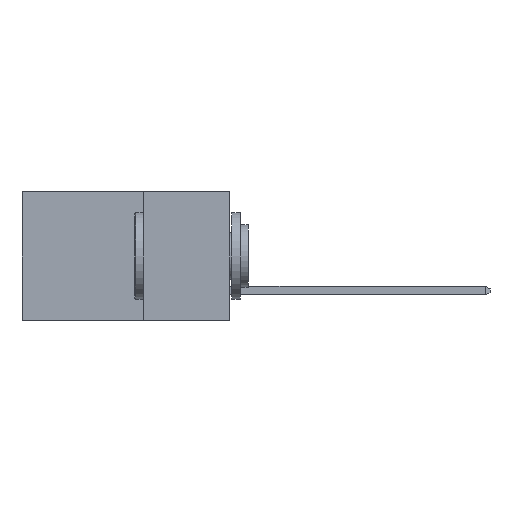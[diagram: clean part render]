
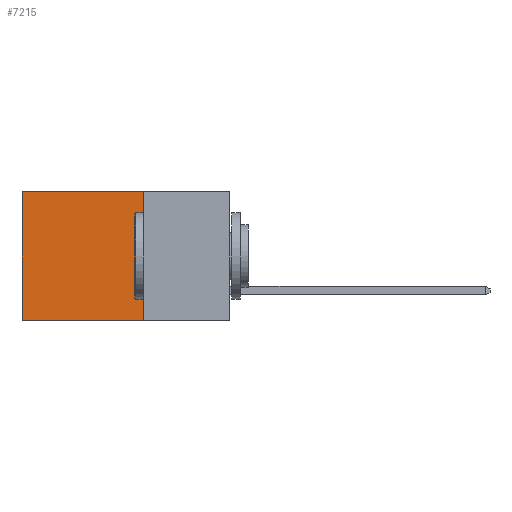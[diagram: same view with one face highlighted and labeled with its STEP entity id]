
A CAD part, left-side view. The second image highlights one B-rep face of the part: STEP entity #7215.
In plain terms, the highlighted planar face has unit normal (-1, 0, 0).
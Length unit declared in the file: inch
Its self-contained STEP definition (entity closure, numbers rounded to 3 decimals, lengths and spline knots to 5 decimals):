
#137 = VERTEX_POINT ( 'NONE', #3383 ) ;
#369 = EDGE_CURVE ( 'NONE', #3417, #3736, #3243, .T. ) ;
#372 = CARTESIAN_POINT ( 'NONE',  ( 0.2615, 0.25, -0.37 ) ) ;
#1125 = LINE ( 'NONE', #10935, #9800 ) ;
#3243 = LINE ( 'NONE', #10252, #4630 ) ;
#3383 = CARTESIAN_POINT ( 'NONE',  ( 0.2615, 0.6, 0. ) ) ;
#3417 = VERTEX_POINT ( 'NONE', #372 ) ;
#3736 = VERTEX_POINT ( 'NONE', #4516 ) ;
#3768 = FACE_OUTER_BOUND ( 'NONE', #9711, .T. ) ;
#4274 = DIRECTION ( 'NONE',  ( 0., 0., -1. ) ) ;
#4364 = ORIENTED_EDGE ( 'NONE', *, *, #12494, .T. ) ;
#4516 = CARTESIAN_POINT ( 'NONE',  ( 0.2615, 0.6, -0.37 ) ) ;
#4630 = VECTOR ( 'NONE', #11599, 39.37008 ) ;
#4974 = AXIS2_PLACEMENT_3D ( 'NONE', #5046, #10519, #7275 ) ;
#5046 = CARTESIAN_POINT ( 'NONE',  ( 0.2615, 0.25, -0.37 ) ) ;
#7215 = ADVANCED_FACE ( 'NONE', ( #3768 ), #11588, .F. ) ;
#7275 = DIRECTION ( 'NONE',  ( 0., 0., -1. ) ) ;
#7659 = VECTOR ( 'NONE', #11842, 39.37008 ) ;
#8395 = DIRECTION ( 'NONE',  ( 0., 1., 0. ) ) ;
#8411 = ORIENTED_EDGE ( 'NONE', *, *, #13569, .T. ) ;
#9667 = CARTESIAN_POINT ( 'NONE',  ( 0.2615, 0.25, -0.37 ) ) ;
#9711 = EDGE_LOOP ( 'NONE', ( #8411, #11361, #12834, #4364 ) ) ;
#9800 = VECTOR ( 'NONE', #4274, 39.37008 ) ;
#10252 = CARTESIAN_POINT ( 'NONE',  ( 0.2615, 0.25, -0.37 ) ) ;
#10519 = DIRECTION ( 'NONE',  ( 1., 0., 0. ) ) ;
#10717 = CARTESIAN_POINT ( 'NONE',  ( 0.2615, 0.25, 0. ) ) ;
#10809 = EDGE_CURVE ( 'NONE', #10903, #3417, #12602, .T. ) ;
#10903 = VERTEX_POINT ( 'NONE', #10717 ) ;
#10935 = CARTESIAN_POINT ( 'NONE',  ( 0.2615, 0.6, -0.37 ) ) ;
#11357 = LINE ( 'NONE', #12829, #12722 ) ;
#11361 = ORIENTED_EDGE ( 'NONE', *, *, #369, .F. ) ;
#11588 = PLANE ( 'NONE',  #4974 ) ;
#11599 = DIRECTION ( 'NONE',  ( 0., 1., 0. ) ) ;
#11842 = DIRECTION ( 'NONE',  ( 0., 0., -1. ) ) ;
#12494 = EDGE_CURVE ( 'NONE', #10903, #137, #11357, .T. ) ;
#12602 = LINE ( 'NONE', #9667, #7659 ) ;
#12722 = VECTOR ( 'NONE', #8395, 39.37008 ) ;
#12829 = CARTESIAN_POINT ( 'NONE',  ( 0.2615, 0.25, 0. ) ) ;
#12834 = ORIENTED_EDGE ( 'NONE', *, *, #10809, .F. ) ;
#13569 = EDGE_CURVE ( 'NONE', #137, #3736, #1125, .T. ) ;
